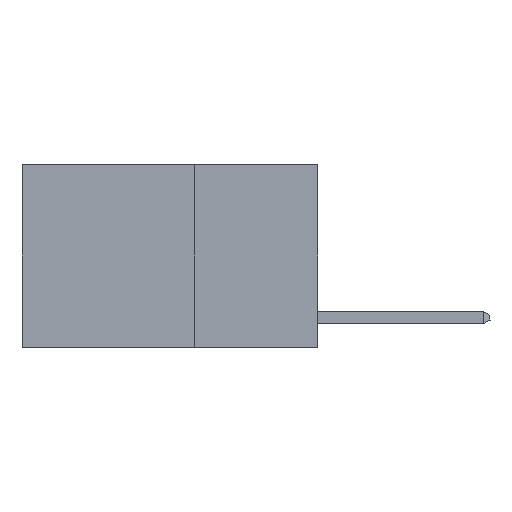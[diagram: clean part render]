
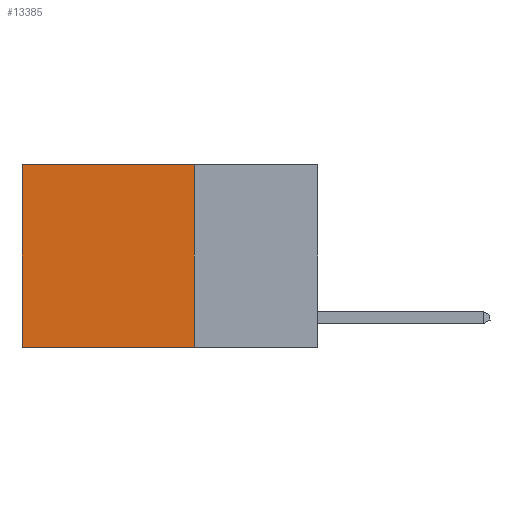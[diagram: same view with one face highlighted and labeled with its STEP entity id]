
A CAD part, left-side view. The second image highlights one B-rep face of the part: STEP entity #13385.
In plain terms, the highlighted planar face has unit normal (-1, 0, 0).
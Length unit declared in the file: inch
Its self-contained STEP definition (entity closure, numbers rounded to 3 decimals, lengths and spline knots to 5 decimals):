
#617 = CARTESIAN_POINT ( 'NONE',  ( 0.2625, 0.25, 0. ) ) ;
#1695 = ORIENTED_EDGE ( 'NONE', *, *, #14534, .F. ) ;
#1794 = CARTESIAN_POINT ( 'NONE',  ( 0.2625, 0.6, 0. ) ) ;
#2288 = VECTOR ( 'NONE', #20502, 39.37008 ) ;
#3021 = DIRECTION ( 'NONE',  ( 0., 0., -1. ) ) ;
#3456 = LINE ( 'NONE', #9655, #20742 ) ;
#4481 = EDGE_CURVE ( 'NONE', #15634, #16381, #18265, .T. ) ;
#4881 = VECTOR ( 'NONE', #17458, 39.37008 ) ;
#5718 = CARTESIAN_POINT ( 'NONE',  ( 0.2625, 0.25, -0.37 ) ) ;
#6113 = CARTESIAN_POINT ( 'NONE',  ( 0.2625, 0.25, -0.37 ) ) ;
#6897 = VERTEX_POINT ( 'NONE', #1794 ) ;
#8464 = DIRECTION ( 'NONE',  ( 1., 0., 0. ) ) ;
#8723 = FACE_OUTER_BOUND ( 'NONE', #18804, .T. ) ;
#9655 = CARTESIAN_POINT ( 'NONE',  ( 0.2625, 0.25, 0. ) ) ;
#10658 = LINE ( 'NONE', #13828, #2288 ) ;
#11272 = VERTEX_POINT ( 'NONE', #617 ) ;
#11299 = ORIENTED_EDGE ( 'NONE', *, *, #4481, .F. ) ;
#11688 = DIRECTION ( 'NONE',  ( 0., 0., -1. ) ) ;
#11994 = CARTESIAN_POINT ( 'NONE',  ( 0.2625, 0.6, -0.37 ) ) ;
#12141 = LINE ( 'NONE', #21709, #21059 ) ;
#13369 = PLANE ( 'NONE',  #13873 ) ;
#13385 = ADVANCED_FACE ( 'NONE', ( #8723 ), #13369, .F. ) ;
#13828 = CARTESIAN_POINT ( 'NONE',  ( 0.2625, 0.25, 0. ) ) ;
#13873 = AXIS2_PLACEMENT_3D ( 'NONE', #18534, #8464, #20199 ) ;
#14534 = EDGE_CURVE ( 'NONE', #11272, #15634, #3456, .T. ) ;
#15634 = VERTEX_POINT ( 'NONE', #6113 ) ;
#16381 = VERTEX_POINT ( 'NONE', #11994 ) ;
#17458 = DIRECTION ( 'NONE',  ( 0., 1., 0. ) ) ;
#18265 = LINE ( 'NONE', #5718, #4881 ) ;
#18534 = CARTESIAN_POINT ( 'NONE',  ( 0.2625, 0.25, 0. ) ) ;
#18804 = EDGE_LOOP ( 'NONE', ( #20425, #11299, #1695, #20495 ) ) ;
#19170 = EDGE_CURVE ( 'NONE', #11272, #6897, #10658, .T. ) ;
#20199 = DIRECTION ( 'NONE',  ( 0., 0., -1. ) ) ;
#20425 = ORIENTED_EDGE ( 'NONE', *, *, #20809, .T. ) ;
#20495 = ORIENTED_EDGE ( 'NONE', *, *, #19170, .T. ) ;
#20502 = DIRECTION ( 'NONE',  ( 0., 1., 0. ) ) ;
#20742 = VECTOR ( 'NONE', #3021, 39.37008 ) ;
#20809 = EDGE_CURVE ( 'NONE', #6897, #16381, #12141, .T. ) ;
#21059 = VECTOR ( 'NONE', #11688, 39.37008 ) ;
#21709 = CARTESIAN_POINT ( 'NONE',  ( 0.2625, 0.6, 0. ) ) ;
